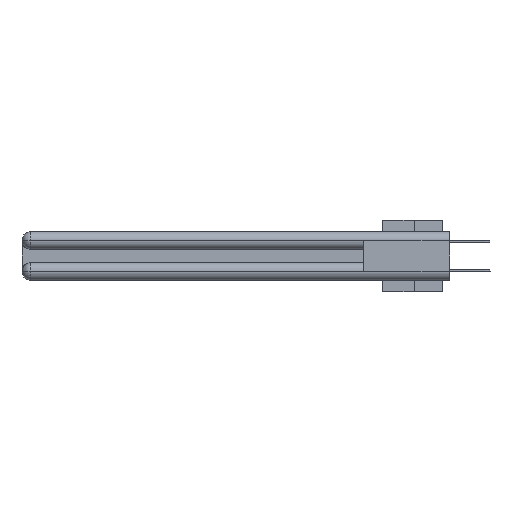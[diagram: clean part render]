
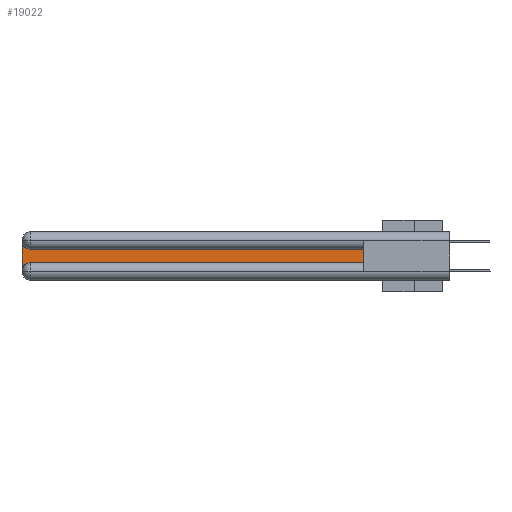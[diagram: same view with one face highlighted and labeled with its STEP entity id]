
A CAD part, left-side view. The second image highlights one B-rep face of the part: STEP entity #19022.
In plain terms, the highlighted planar face has unit normal (-1, 0, 0).
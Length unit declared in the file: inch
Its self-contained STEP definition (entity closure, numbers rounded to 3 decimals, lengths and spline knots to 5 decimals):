
#463 = CIRCLE ( 'NONE', #9504, 0.06 ) ;
#1033 = CARTESIAN_POINT ( 'NONE',  ( 0.075, 0.6, -0.2175 ) ) ;
#1748 = CARTESIAN_POINT ( 'NONE',  ( 0.075, 0.6, -0.1225 ) ) ;
#4193 = DIRECTION ( 'NONE',  ( 1., 0., 0. ) ) ;
#4618 = VECTOR ( 'NONE', #8153, 39.37008 ) ;
#5347 = DIRECTION ( 'NONE',  ( 1., 0., 0. ) ) ;
#6904 = LINE ( 'NONE', #29319, #9843 ) ;
#7024 = CARTESIAN_POINT ( 'NONE',  ( 0.075, 3., -0.1225 ) ) ;
#7137 = VERTEX_POINT ( 'NONE', #23811 ) ;
#8051 = AXIS2_PLACEMENT_3D ( 'NONE', #7024, #4193, #33407 ) ;
#8153 = DIRECTION ( 'NONE',  ( 0., -1., 0. ) ) ;
#8384 = CARTESIAN_POINT ( 'NONE',  ( 0.075, 2.94, -0.2175 ) ) ;
#8394 = EDGE_CURVE ( 'NONE', #11969, #23615, #6904, .T. ) ;
#9504 = AXIS2_PLACEMENT_3D ( 'NONE', #31145, #34255, #31602 ) ;
#9843 = VECTOR ( 'NONE', #13200, 39.37008 ) ;
#11635 = ORIENTED_EDGE ( 'NONE', *, *, #12674, .T. ) ;
#11969 = VERTEX_POINT ( 'NONE', #1033 ) ;
#12543 = ORIENTED_EDGE ( 'NONE', *, *, #27015, .T. ) ;
#12674 = EDGE_CURVE ( 'NONE', #7137, #29310, #463, .T. ) ;
#13027 = ORIENTED_EDGE ( 'NONE', *, *, #21603, .T. ) ;
#13200 = DIRECTION ( 'NONE',  ( 0., 0., 1. ) ) ;
#13404 = VECTOR ( 'NONE', #14985, 39.37008 ) ;
#14117 = AXIS2_PLACEMENT_3D ( 'NONE', #15806, #5347, #18242 ) ;
#14985 = DIRECTION ( 'NONE',  ( 0., 0., -1. ) ) ;
#15806 = CARTESIAN_POINT ( 'NONE',  ( 0.075, 2.94, -0.0625 ) ) ;
#15822 = ORIENTED_EDGE ( 'NONE', *, *, #8394, .T. ) ;
#17617 = CARTESIAN_POINT ( 'NONE',  ( 0.075, 0.6, -0.1225 ) ) ;
#18242 = DIRECTION ( 'NONE',  ( 0., 0., -1. ) ) ;
#19022 = ADVANCED_FACE ( 'NONE', ( #21081 ), #22712, .F. ) ;
#20922 = LINE ( 'NONE', #22815, #13404 ) ;
#21081 = FACE_OUTER_BOUND ( 'NONE', #31543, .T. ) ;
#21266 = CARTESIAN_POINT ( 'NONE',  ( 0.075, 0.6, -0.2175 ) ) ;
#21603 = EDGE_CURVE ( 'NONE', #23615, #33130, #26768, .T. ) ;
#22712 = PLANE ( 'NONE',  #8051 ) ;
#22815 = CARTESIAN_POINT ( 'NONE',  ( 0.075, 3., -0.2175 ) ) ;
#23615 = VERTEX_POINT ( 'NONE', #17617 ) ;
#23811 = CARTESIAN_POINT ( 'NONE',  ( 0.075, 3., -0.2775 ) ) ;
#26768 = LINE ( 'NONE', #1748, #27998 ) ;
#26868 = CARTESIAN_POINT ( 'NONE',  ( 0.075, 3., -0.0625 ) ) ;
#27015 = EDGE_CURVE ( 'NONE', #30499, #7137, #20922, .T. ) ;
#27875 = EDGE_CURVE ( 'NONE', #29310, #11969, #33866, .T. ) ;
#27998 = VECTOR ( 'NONE', #28645, 39.37008 ) ;
#28380 = CIRCLE ( 'NONE', #14117, 0.06 ) ;
#28645 = DIRECTION ( 'NONE',  ( 0., 1., 0. ) ) ;
#29310 = VERTEX_POINT ( 'NONE', #8384 ) ;
#29319 = CARTESIAN_POINT ( 'NONE',  ( 0.075, 0.6, -0.2175 ) ) ;
#30337 = EDGE_CURVE ( 'NONE', #33130, #30499, #28380, .T. ) ;
#30499 = VERTEX_POINT ( 'NONE', #26868 ) ;
#31145 = CARTESIAN_POINT ( 'NONE',  ( 0.075, 2.94, -0.2775 ) ) ;
#31543 = EDGE_LOOP ( 'NONE', ( #13027, #32243, #12543, #11635, #32490, #15822 ) ) ;
#31602 = DIRECTION ( 'NONE',  ( 0., 0., -1. ) ) ;
#32243 = ORIENTED_EDGE ( 'NONE', *, *, #30337, .T. ) ;
#32490 = ORIENTED_EDGE ( 'NONE', *, *, #27875, .T. ) ;
#32603 = CARTESIAN_POINT ( 'NONE',  ( 0.075, 2.94, -0.1225 ) ) ;
#33130 = VERTEX_POINT ( 'NONE', #32603 ) ;
#33407 = DIRECTION ( 'NONE',  ( 0., 0., -1. ) ) ;
#33866 = LINE ( 'NONE', #21266, #4618 ) ;
#34255 = DIRECTION ( 'NONE',  ( 1., 0., 0. ) ) ;
